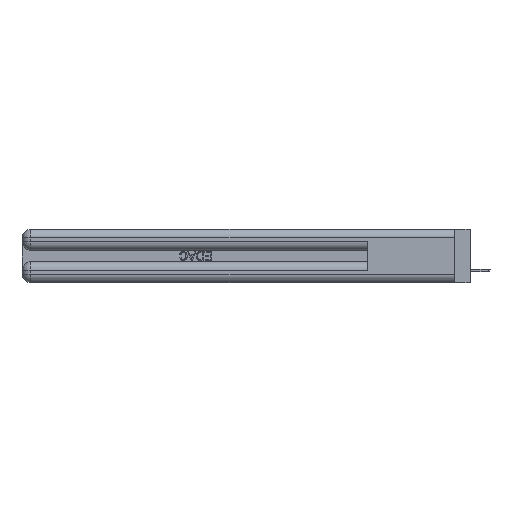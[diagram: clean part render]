
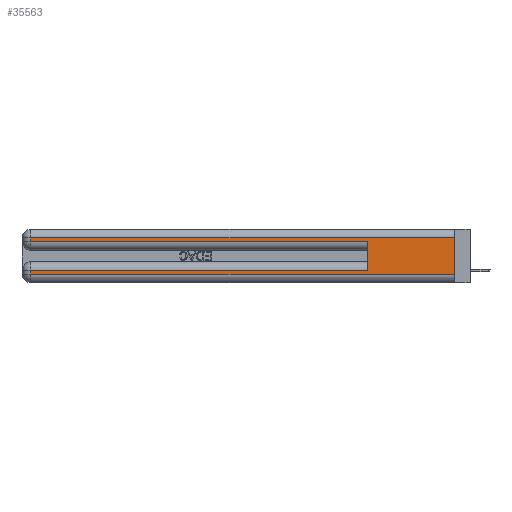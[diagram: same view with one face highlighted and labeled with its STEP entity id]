
A CAD part, left-side view. The second image highlights one B-rep face of the part: STEP entity #35563.
In plain terms, the highlighted planar face has unit normal (-1, 0, 0).
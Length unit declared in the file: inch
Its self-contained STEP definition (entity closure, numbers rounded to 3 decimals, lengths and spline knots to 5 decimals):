
#1106 = CARTESIAN_POINT ( 'NONE',  ( 0., 0., 0.31 ) ) ;
#3792 = LINE ( 'NONE', #7366, #22221 ) ;
#3818 = EDGE_CURVE ( 'NONE', #25117, #12654, #6138, .T. ) ;
#4806 = EDGE_CURVE ( 'NONE', #23952, #27553, #3792, .T. ) ;
#5985 = FACE_OUTER_BOUND ( 'NONE', #38892, .T. ) ;
#6009 = DIRECTION ( 'NONE',  ( 0., 0., 1. ) ) ;
#6138 = LINE ( 'NONE', #16257, #43071 ) ;
#6246 = ORIENTED_EDGE ( 'NONE', *, *, #4806, .F. ) ;
#6900 = CARTESIAN_POINT ( 'NONE',  ( 0., 0.6, 0.145 ) ) ;
#7032 = DIRECTION ( 'NONE',  ( 0., -1., 0. ) ) ;
#7045 = EDGE_CURVE ( 'NONE', #22372, #27553, #44376, .T. ) ;
#7366 = CARTESIAN_POINT ( 'NONE',  ( 0., 0., 0.37 ) ) ;
#7551 = VERTEX_POINT ( 'NONE', #11954 ) ;
#7847 = DIRECTION ( 'NONE',  ( 0., 1., 0. ) ) ;
#8757 = ORIENTED_EDGE ( 'NONE', *, *, #38862, .T. ) ;
#10083 = AXIS2_PLACEMENT_3D ( 'NONE', #32758, #12318, #33419 ) ;
#10420 = LINE ( 'NONE', #34691, #25325 ) ;
#11954 = CARTESIAN_POINT ( 'NONE',  ( 0., 2.94, 0.285 ) ) ;
#12318 = DIRECTION ( 'NONE',  ( 1., 0., 0. ) ) ;
#12654 = VERTEX_POINT ( 'NONE', #37389 ) ;
#12716 = EDGE_CURVE ( 'NONE', #7551, #23887, #10420, .T. ) ;
#13411 = ORIENTED_EDGE ( 'NONE', *, *, #40893, .T. ) ;
#13824 = LINE ( 'NONE', #38508, #30666 ) ;
#14212 = CARTESIAN_POINT ( 'NONE',  ( 0., 2.94, 0.31 ) ) ;
#14618 = EDGE_CURVE ( 'NONE', #15737, #7551, #21964, .T. ) ;
#15049 = LINE ( 'NONE', #1106, #33687 ) ;
#15737 = VERTEX_POINT ( 'NONE', #14212 ) ;
#16257 = CARTESIAN_POINT ( 'NONE',  ( 0., 0., 0.085 ) ) ;
#18129 = ORIENTED_EDGE ( 'NONE', *, *, #39454, .F. ) ;
#19716 = PLANE ( 'NONE',  #10083 ) ;
#19875 = DIRECTION ( 'NONE',  ( 0., 1., 0. ) ) ;
#20490 = VECTOR ( 'NONE', #23257, 39.37008 ) ;
#20625 = LINE ( 'NONE', #6900, #29284 ) ;
#21964 = LINE ( 'NONE', #32967, #26869 ) ;
#22221 = VECTOR ( 'NONE', #44255, 39.37008 ) ;
#22260 = ORIENTED_EDGE ( 'NONE', *, *, #7045, .T. ) ;
#22372 = VERTEX_POINT ( 'NONE', #39799 ) ;
#22448 = CARTESIAN_POINT ( 'NONE',  ( 0., 0.6, 0.285 ) ) ;
#23257 = DIRECTION ( 'NONE',  ( 0., -1., 0. ) ) ;
#23887 = VERTEX_POINT ( 'NONE', #22448 ) ;
#23952 = VERTEX_POINT ( 'NONE', #36143 ) ;
#25117 = VERTEX_POINT ( 'NONE', #42900 ) ;
#25325 = VECTOR ( 'NONE', #7032, 39.37008 ) ;
#25783 = DIRECTION ( 'NONE',  ( 0., 0., -1. ) ) ;
#26869 = VECTOR ( 'NONE', #25783, 39.37008 ) ;
#27512 = DIRECTION ( 'NONE',  ( 0., 0., -1. ) ) ;
#27553 = VERTEX_POINT ( 'NONE', #44227 ) ;
#29284 = VECTOR ( 'NONE', #6009, 39.37008 ) ;
#30666 = VECTOR ( 'NONE', #27512, 39.37008 ) ;
#32758 = CARTESIAN_POINT ( 'NONE',  ( 0., 0., 0.37 ) ) ;
#32967 = CARTESIAN_POINT ( 'NONE',  ( 0., 2.94, 0.37 ) ) ;
#33419 = DIRECTION ( 'NONE',  ( 0., 0., -1. ) ) ;
#33687 = VECTOR ( 'NONE', #7847, 39.37008 ) ;
#34691 = CARTESIAN_POINT ( 'NONE',  ( 0., 0., 0.285 ) ) ;
#35563 = ADVANCED_FACE ( 'NONE', ( #5985 ), #19716, .F. ) ;
#36143 = CARTESIAN_POINT ( 'NONE',  ( 0., 0., 0.31 ) ) ;
#37389 = CARTESIAN_POINT ( 'NONE',  ( 0., 2.94, 0.085 ) ) ;
#37761 = ORIENTED_EDGE ( 'NONE', *, *, #14618, .T. ) ;
#37833 = CARTESIAN_POINT ( 'NONE',  ( 0., 0., 0.06 ) ) ;
#38508 = CARTESIAN_POINT ( 'NONE',  ( 0., 2.94, 0.37 ) ) ;
#38862 = EDGE_CURVE ( 'NONE', #12654, #22372, #13824, .T. ) ;
#38892 = EDGE_LOOP ( 'NONE', ( #6246, #13411, #37761, #41208, #18129, #41929, #8757, #22260 ) ) ;
#39454 = EDGE_CURVE ( 'NONE', #25117, #23887, #20625, .T. ) ;
#39799 = CARTESIAN_POINT ( 'NONE',  ( 0., 2.94, 0.06 ) ) ;
#40893 = EDGE_CURVE ( 'NONE', #23952, #15737, #15049, .T. ) ;
#41208 = ORIENTED_EDGE ( 'NONE', *, *, #12716, .T. ) ;
#41929 = ORIENTED_EDGE ( 'NONE', *, *, #3818, .T. ) ;
#42900 = CARTESIAN_POINT ( 'NONE',  ( 0., 0.6, 0.085 ) ) ;
#43071 = VECTOR ( 'NONE', #19875, 39.37008 ) ;
#44227 = CARTESIAN_POINT ( 'NONE',  ( 0., 0., 0.06 ) ) ;
#44255 = DIRECTION ( 'NONE',  ( 0., 0., -1. ) ) ;
#44376 = LINE ( 'NONE', #37833, #20490 ) ;
